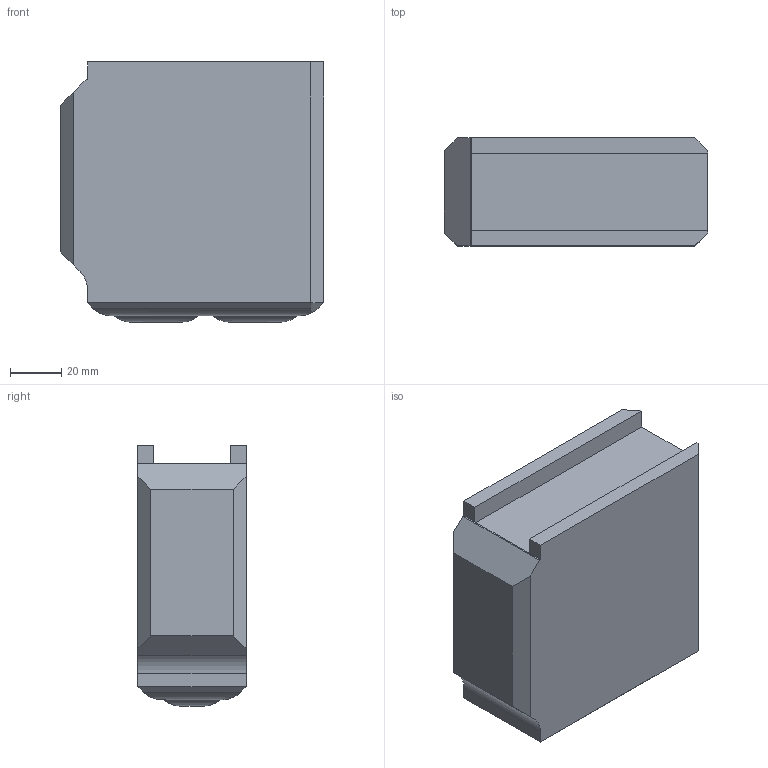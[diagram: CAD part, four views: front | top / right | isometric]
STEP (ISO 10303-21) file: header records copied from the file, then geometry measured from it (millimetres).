
FILE_DESCRIPTION (( 'STEP AP214' ), '1' );
FILE_NAME ('hydrastocky3.STEP', '2013-07-04T02:36:38', ( '' ), ( '' ), 'SwSTEP 2.0', 'SolidWorks 2012', '' );
FILE_SCHEMA (( 'AUTOMOTIVE_DESIGN' ));
Length unit declared in the file: inch
Products named in the file (1): hydrastocky3
Bounding box: 102.51 x 42.16 x 101.39 mm (x, y, z)
Volume: 387444.6 mm3; surface area: 35257.2 mm2
Topology: 1 solids, 1 shells, 42 faces, 104 edges, 66 vertices
Faces by surface type: plane 29, cylinder 13
Entity records: 1250 total; most frequent: CARTESIAN_POINT 261, ORIENTED_EDGE 208, DIRECTION 176, EDGE_CURVE 104, VECTOR 86, LINE 86, VERTEX_POINT 66, AXIS2_PLACEMENT_3D 45
